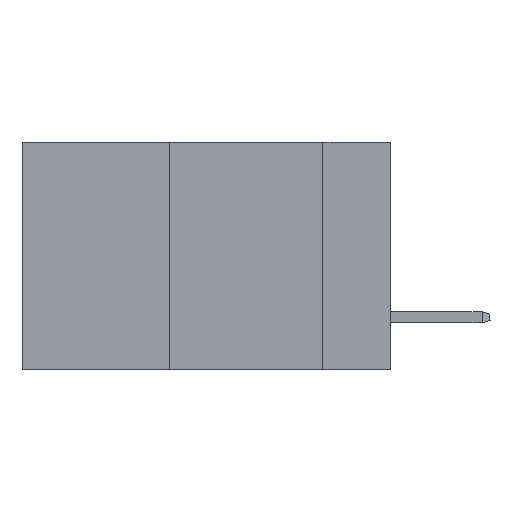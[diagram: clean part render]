
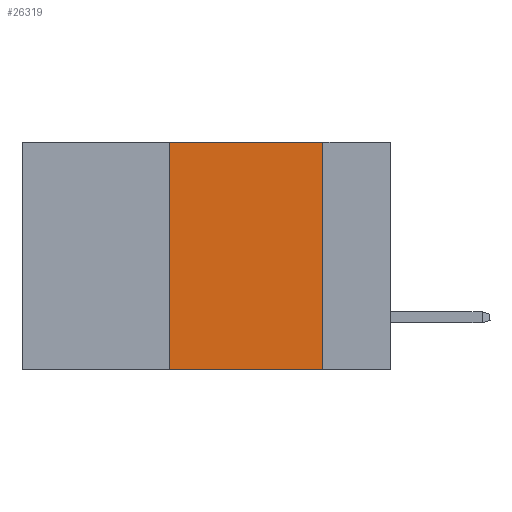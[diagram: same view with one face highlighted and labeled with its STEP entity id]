
A CAD part, left-side view. The second image highlights one B-rep face of the part: STEP entity #26319.
In plain terms, the highlighted planar face has unit normal (-1, 0, 0).
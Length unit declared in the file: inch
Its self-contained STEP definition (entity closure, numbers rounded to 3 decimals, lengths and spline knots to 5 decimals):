
#859 = LINE ( 'NONE', #8287, #13845 ) ;
#1587 = DIRECTION ( 'NONE',  ( 1., 0., 0. ) ) ;
#1984 = DIRECTION ( 'NONE',  ( 0., 0., -1. ) ) ;
#3293 = VECTOR ( 'NONE', #1984, 39.37008 ) ;
#3731 = EDGE_CURVE ( 'NONE', #12604, #32027, #13213, .T. ) ;
#7428 = ORIENTED_EDGE ( 'NONE', *, *, #14738, .F. ) ;
#7682 = ORIENTED_EDGE ( 'NONE', *, *, #23516, .T. ) ;
#8287 = CARTESIAN_POINT ( 'NONE',  ( 0., 0.6, -0.37 ) ) ;
#9222 = LINE ( 'NONE', #43318, #3293 ) ;
#10504 = EDGE_CURVE ( 'NONE', #44240, #12604, #36757, .T. ) ;
#11531 = CARTESIAN_POINT ( 'NONE',  ( 0., 0.6, 0. ) ) ;
#12604 = VERTEX_POINT ( 'NONE', #39451 ) ;
#13213 = LINE ( 'NONE', #36043, #36419 ) ;
#13845 = VECTOR ( 'NONE', #25341, 39.37008 ) ;
#14738 = EDGE_CURVE ( 'NONE', #32027, #30076, #9222, .T. ) ;
#15313 = PLANE ( 'NONE',  #27328 ) ;
#17382 = FACE_OUTER_BOUND ( 'NONE', #35607, .T. ) ;
#20576 = VECTOR ( 'NONE', #31304, 39.37008 ) ;
#23516 = EDGE_CURVE ( 'NONE', #44240, #30076, #859, .T. ) ;
#25341 = DIRECTION ( 'NONE',  ( 0., -1., 0. ) ) ;
#26319 = ADVANCED_FACE ( 'NONE', ( #17382 ), #15313, .F. ) ;
#27328 = AXIS2_PLACEMENT_3D ( 'NONE', #11531, #1587, #32361 ) ;
#28635 = DIRECTION ( 'NONE',  ( 0., -1., 0. ) ) ;
#29114 = CARTESIAN_POINT ( 'NONE',  ( 0., 0.36, -0.37 ) ) ;
#30076 = VERTEX_POINT ( 'NONE', #40211 ) ;
#31304 = DIRECTION ( 'NONE',  ( 0., 0., 1. ) ) ;
#32027 = VERTEX_POINT ( 'NONE', #33266 ) ;
#32361 = DIRECTION ( 'NONE',  ( 0., 0., -1. ) ) ;
#33266 = CARTESIAN_POINT ( 'NONE',  ( 0., 0.11, 0. ) ) ;
#35058 = CARTESIAN_POINT ( 'NONE',  ( 0., 0.36, 0. ) ) ;
#35607 = EDGE_LOOP ( 'NONE', ( #7428, #39356, #36648, #7682 ) ) ;
#36043 = CARTESIAN_POINT ( 'NONE',  ( 0., 0.6, 0. ) ) ;
#36419 = VECTOR ( 'NONE', #28635, 39.37008 ) ;
#36648 = ORIENTED_EDGE ( 'NONE', *, *, #10504, .F. ) ;
#36757 = LINE ( 'NONE', #35058, #20576 ) ;
#39356 = ORIENTED_EDGE ( 'NONE', *, *, #3731, .F. ) ;
#39451 = CARTESIAN_POINT ( 'NONE',  ( 0., 0.36, 0. ) ) ;
#40211 = CARTESIAN_POINT ( 'NONE',  ( 0., 0.11, -0.37 ) ) ;
#43318 = CARTESIAN_POINT ( 'NONE',  ( 0., 0.11, 0. ) ) ;
#44240 = VERTEX_POINT ( 'NONE', #29114 ) ;
